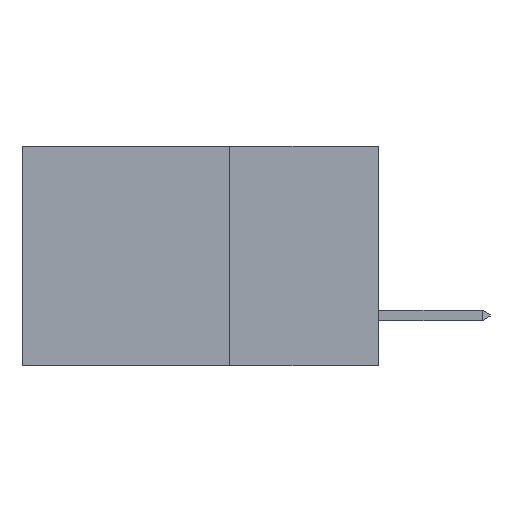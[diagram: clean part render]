
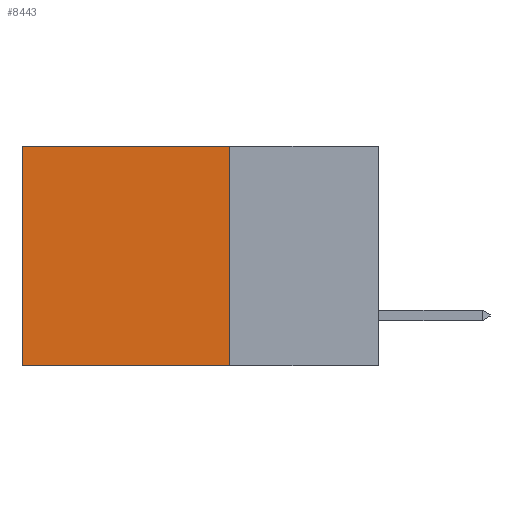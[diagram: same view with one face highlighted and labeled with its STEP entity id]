
A CAD part, left-side view. The second image highlights one B-rep face of the part: STEP entity #8443.
In plain terms, the highlighted planar face has unit normal (-1, 0, 0).
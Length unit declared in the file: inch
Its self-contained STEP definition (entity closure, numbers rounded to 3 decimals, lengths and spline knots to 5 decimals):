
#270 = VERTEX_POINT ( 'NONE', #9467 ) ;
#585 = EDGE_CURVE ( 'NONE', #8776, #9212, #1250, .T. ) ;
#1250 = LINE ( 'NONE', #3972, #14020 ) ;
#1890 = CARTESIAN_POINT ( 'NONE',  ( 0.298, 0.25, 0. ) ) ;
#2635 = ORIENTED_EDGE ( 'NONE', *, *, #13780, .F. ) ;
#3186 = DIRECTION ( 'NONE',  ( 0., 0., -1. ) ) ;
#3213 = EDGE_CURVE ( 'NONE', #270, #8776, #10643, .T. ) ;
#3368 = EDGE_LOOP ( 'NONE', ( #14185, #2635, #10120, #8141 ) ) ;
#3810 = EDGE_CURVE ( 'NONE', #270, #15577, #15080, .T. ) ;
#3972 = CARTESIAN_POINT ( 'NONE',  ( 0.298, 0.6, 0. ) ) ;
#6957 = DIRECTION ( 'NONE',  ( 0., 0., -1. ) ) ;
#7347 = VECTOR ( 'NONE', #12361, 39.37008 ) ;
#8130 = PLANE ( 'NONE',  #8957 ) ;
#8141 = ORIENTED_EDGE ( 'NONE', *, *, #3213, .T. ) ;
#8399 = CARTESIAN_POINT ( 'NONE',  ( 0.298, 0.25, -0.37 ) ) ;
#8443 = ADVANCED_FACE ( 'NONE', ( #14853 ), #8130, .F. ) ;
#8654 = LINE ( 'NONE', #10989, #11933 ) ;
#8776 = VERTEX_POINT ( 'NONE', #11215 ) ;
#8788 = CARTESIAN_POINT ( 'NONE',  ( 0.298, 0.25, 0. ) ) ;
#8957 = AXIS2_PLACEMENT_3D ( 'NONE', #1890, #10638, #3186 ) ;
#9212 = VERTEX_POINT ( 'NONE', #14312 ) ;
#9467 = CARTESIAN_POINT ( 'NONE',  ( 0.298, 0.25, 0. ) ) ;
#10120 = ORIENTED_EDGE ( 'NONE', *, *, #3810, .F. ) ;
#10191 = DIRECTION ( 'NONE',  ( 0., 0., -1. ) ) ;
#10638 = DIRECTION ( 'NONE',  ( 1., 0., 0. ) ) ;
#10643 = LINE ( 'NONE', #15318, #7347 ) ;
#10989 = CARTESIAN_POINT ( 'NONE',  ( 0.298, 0.25, -0.37 ) ) ;
#11215 = CARTESIAN_POINT ( 'NONE',  ( 0.298, 0.6, 0. ) ) ;
#11933 = VECTOR ( 'NONE', #15690, 39.37008 ) ;
#11954 = VECTOR ( 'NONE', #10191, 39.37008 ) ;
#12361 = DIRECTION ( 'NONE',  ( 0., 1., 0. ) ) ;
#13780 = EDGE_CURVE ( 'NONE', #15577, #9212, #8654, .T. ) ;
#14020 = VECTOR ( 'NONE', #6957, 39.37008 ) ;
#14185 = ORIENTED_EDGE ( 'NONE', *, *, #585, .T. ) ;
#14312 = CARTESIAN_POINT ( 'NONE',  ( 0.298, 0.6, -0.37 ) ) ;
#14853 = FACE_OUTER_BOUND ( 'NONE', #3368, .T. ) ;
#15080 = LINE ( 'NONE', #8788, #11954 ) ;
#15318 = CARTESIAN_POINT ( 'NONE',  ( 0.298, 0.25, 0. ) ) ;
#15577 = VERTEX_POINT ( 'NONE', #8399 ) ;
#15690 = DIRECTION ( 'NONE',  ( 0., 1., 0. ) ) ;
